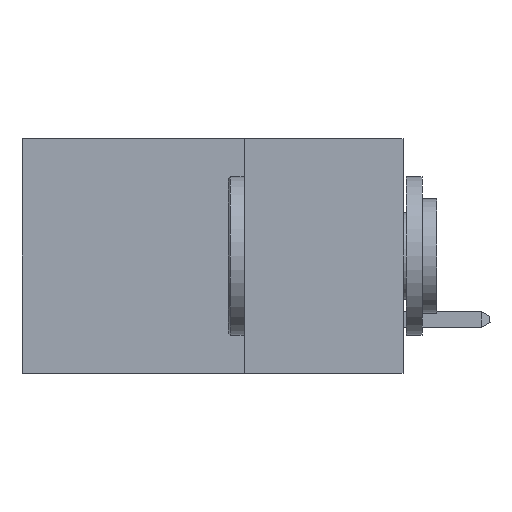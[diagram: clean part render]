
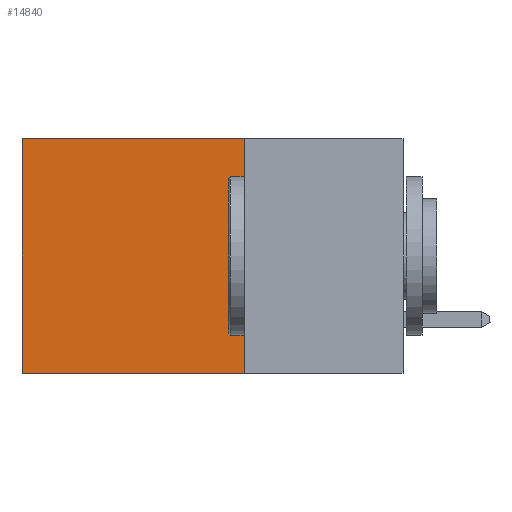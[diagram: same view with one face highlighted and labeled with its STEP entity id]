
A CAD part, left-side view. The second image highlights one B-rep face of the part: STEP entity #14840.
In plain terms, the highlighted planar face has unit normal (-1, 0, 0).
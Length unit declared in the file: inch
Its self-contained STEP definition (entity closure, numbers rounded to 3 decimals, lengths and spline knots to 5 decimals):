
#187 = VECTOR ( 'NONE', #9189, 39.37008 ) ;
#548 = VECTOR ( 'NONE', #12828, 39.37008 ) ;
#799 = CARTESIAN_POINT ( 'NONE',  ( 0.2875, 0.6, 0. ) ) ;
#2195 = CARTESIAN_POINT ( 'NONE',  ( 0.2875, 0.6, 0. ) ) ;
#2386 = VECTOR ( 'NONE', #14287, 39.37008 ) ;
#2730 = DIRECTION ( 'NONE',  ( 0., 1., 0. ) ) ;
#3466 = EDGE_CURVE ( 'NONE', #13596, #4927, #12797, .T. ) ;
#3789 = EDGE_CURVE ( 'NONE', #9163, #13026, #6043, .T. ) ;
#4295 = DIRECTION ( 'NONE',  ( 1., 0., 0. ) ) ;
#4927 = VERTEX_POINT ( 'NONE', #7141 ) ;
#5050 = CARTESIAN_POINT ( 'NONE',  ( 0.2875, 0.25, 0. ) ) ;
#5497 = DIRECTION ( 'NONE',  ( 0., 0., -1. ) ) ;
#6043 = LINE ( 'NONE', #5050, #15263 ) ;
#6844 = CARTESIAN_POINT ( 'NONE',  ( 0.2875, 0.25, -0.37 ) ) ;
#7141 = CARTESIAN_POINT ( 'NONE',  ( 0.2875, 0.6, -0.37 ) ) ;
#8142 = CARTESIAN_POINT ( 'NONE',  ( 0.2875, 0.25, 0. ) ) ;
#8552 = ORIENTED_EDGE ( 'NONE', *, *, #12839, .F. ) ;
#8813 = LINE ( 'NONE', #2195, #2386 ) ;
#9163 = VERTEX_POINT ( 'NONE', #14398 ) ;
#9189 = DIRECTION ( 'NONE',  ( 0., 1., 0. ) ) ;
#10924 = ORIENTED_EDGE ( 'NONE', *, *, #3466, .F. ) ;
#11240 = AXIS2_PLACEMENT_3D ( 'NONE', #14071, #4295, #5497 ) ;
#11543 = CARTESIAN_POINT ( 'NONE',  ( 0.2875, 0.25, -0.37 ) ) ;
#11603 = PLANE ( 'NONE',  #11240 ) ;
#12461 = EDGE_LOOP ( 'NONE', ( #13208, #10924, #8552, #15447 ) ) ;
#12797 = LINE ( 'NONE', #11543, #187 ) ;
#12828 = DIRECTION ( 'NONE',  ( 0., 0., -1. ) ) ;
#12839 = EDGE_CURVE ( 'NONE', #9163, #13596, #14468, .T. ) ;
#13026 = VERTEX_POINT ( 'NONE', #799 ) ;
#13208 = ORIENTED_EDGE ( 'NONE', *, *, #14285, .T. ) ;
#13486 = FACE_OUTER_BOUND ( 'NONE', #12461, .T. ) ;
#13596 = VERTEX_POINT ( 'NONE', #6844 ) ;
#14071 = CARTESIAN_POINT ( 'NONE',  ( 0.2875, 0.25, 0. ) ) ;
#14285 = EDGE_CURVE ( 'NONE', #13026, #4927, #8813, .T. ) ;
#14287 = DIRECTION ( 'NONE',  ( 0., 0., -1. ) ) ;
#14398 = CARTESIAN_POINT ( 'NONE',  ( 0.2875, 0.25, 0. ) ) ;
#14468 = LINE ( 'NONE', #8142, #548 ) ;
#14840 = ADVANCED_FACE ( 'NONE', ( #13486 ), #11603, .F. ) ;
#15263 = VECTOR ( 'NONE', #2730, 39.37008 ) ;
#15447 = ORIENTED_EDGE ( 'NONE', *, *, #3789, .T. ) ;
